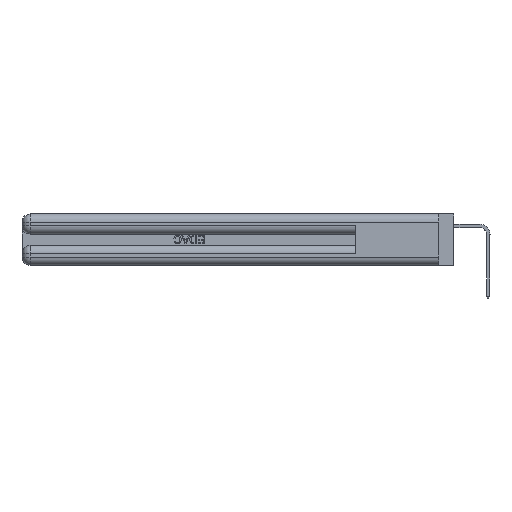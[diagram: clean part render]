
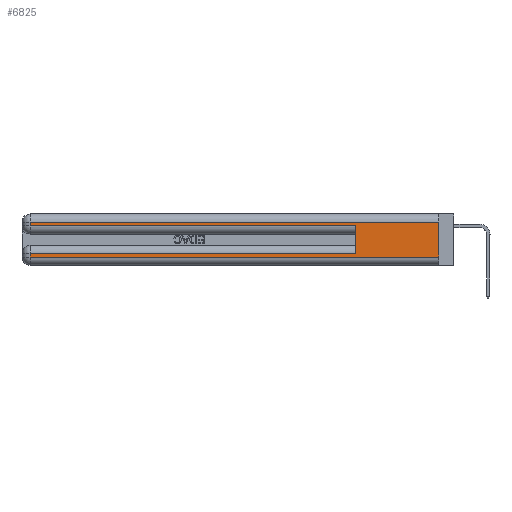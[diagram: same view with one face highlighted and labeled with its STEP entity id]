
A CAD part, left-side view. The second image highlights one B-rep face of the part: STEP entity #6825.
In plain terms, the highlighted planar face has unit normal (-1, 0, 0).
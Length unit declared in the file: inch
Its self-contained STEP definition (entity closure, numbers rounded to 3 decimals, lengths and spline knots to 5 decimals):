
#51 = CARTESIAN_POINT ( 'NONE',  ( 0., 0., 0.31 ) ) ;
#1220 = ORIENTED_EDGE ( 'NONE', *, *, #40643, .T. ) ;
#1501 = LINE ( 'NONE', #16280, #30287 ) ;
#1597 = VECTOR ( 'NONE', #37832, 39.37008 ) ;
#2039 = EDGE_CURVE ( 'NONE', #19701, #25702, #11269, .T. ) ;
#2242 = FACE_OUTER_BOUND ( 'NONE', #19617, .T. ) ;
#2839 = ORIENTED_EDGE ( 'NONE', *, *, #21379, .F. ) ;
#3561 = VERTEX_POINT ( 'NONE', #28904 ) ;
#5607 = PLANE ( 'NONE',  #5820 ) ;
#5661 = LINE ( 'NONE', #15015, #25240 ) ;
#5781 = VECTOR ( 'NONE', #19699, 39.37008 ) ;
#5820 = AXIS2_PLACEMENT_3D ( 'NONE', #48293, #32975, #9551 ) ;
#6825 = ADVANCED_FACE ( 'NONE', ( #2242 ), #5607, .F. ) ;
#7211 = CARTESIAN_POINT ( 'NONE',  ( 0., 0.6, 0.285 ) ) ;
#9551 = DIRECTION ( 'NONE',  ( 0., 0., -1. ) ) ;
#9796 = ORIENTED_EDGE ( 'NONE', *, *, #33480, .T. ) ;
#11269 = LINE ( 'NONE', #28252, #21680 ) ;
#13544 = LINE ( 'NONE', #34298, #42243 ) ;
#14142 = VECTOR ( 'NONE', #47552, 39.37008 ) ;
#15015 = CARTESIAN_POINT ( 'NONE',  ( 0., 2.94, 0.37 ) ) ;
#15180 = EDGE_CURVE ( 'NONE', #19701, #49928, #44286, .T. ) ;
#16280 = CARTESIAN_POINT ( 'NONE',  ( 0., 2.94, 0.37 ) ) ;
#18287 = ORIENTED_EDGE ( 'NONE', *, *, #47482, .T. ) ;
#18958 = DIRECTION ( 'NONE',  ( 0., 0., -1. ) ) ;
#19617 = EDGE_LOOP ( 'NONE', ( #2839, #1220, #26896, #18287, #28642, #39862, #22399, #9796 ) ) ;
#19699 = DIRECTION ( 'NONE',  ( 0., 0., -1. ) ) ;
#19701 = VERTEX_POINT ( 'NONE', #23728 ) ;
#20630 = CARTESIAN_POINT ( 'NONE',  ( 0., 0., 0.31 ) ) ;
#21379 = EDGE_CURVE ( 'NONE', #25191, #44203, #25366, .T. ) ;
#21680 = VECTOR ( 'NONE', #47673, 39.37008 ) ;
#21841 = DIRECTION ( 'NONE',  ( 0., 1., 0. ) ) ;
#22399 = ORIENTED_EDGE ( 'NONE', *, *, #30893, .T. ) ;
#23728 = CARTESIAN_POINT ( 'NONE',  ( 0., 0.6, 0.085 ) ) ;
#25191 = VERTEX_POINT ( 'NONE', #51 ) ;
#25240 = VECTOR ( 'NONE', #18958, 39.37008 ) ;
#25366 = LINE ( 'NONE', #43038, #5781 ) ;
#25702 = VERTEX_POINT ( 'NONE', #7211 ) ;
#26607 = DIRECTION ( 'NONE',  ( 0., -1., 0. ) ) ;
#26896 = ORIENTED_EDGE ( 'NONE', *, *, #31851, .T. ) ;
#28037 = DIRECTION ( 'NONE',  ( 0., 0., -1. ) ) ;
#28252 = CARTESIAN_POINT ( 'NONE',  ( 0., 0.6, 0.145 ) ) ;
#28642 = ORIENTED_EDGE ( 'NONE', *, *, #2039, .F. ) ;
#28904 = CARTESIAN_POINT ( 'NONE',  ( 0., 2.94, 0.06 ) ) ;
#30287 = VECTOR ( 'NONE', #28037, 39.37008 ) ;
#30893 = EDGE_CURVE ( 'NONE', #49928, #3561, #1501, .T. ) ;
#31851 = EDGE_CURVE ( 'NONE', #49597, #37296, #5661, .T. ) ;
#32461 = LINE ( 'NONE', #20630, #14142 ) ;
#32691 = VECTOR ( 'NONE', #21841, 39.37008 ) ;
#32975 = DIRECTION ( 'NONE',  ( 1., 0., 0. ) ) ;
#33480 = EDGE_CURVE ( 'NONE', #3561, #44203, #13544, .T. ) ;
#34298 = CARTESIAN_POINT ( 'NONE',  ( 0., 0., 0.06 ) ) ;
#35158 = CARTESIAN_POINT ( 'NONE',  ( 0., 0., 0.06 ) ) ;
#37296 = VERTEX_POINT ( 'NONE', #37383 ) ;
#37375 = CARTESIAN_POINT ( 'NONE',  ( 0., 0., 0.085 ) ) ;
#37383 = CARTESIAN_POINT ( 'NONE',  ( 0., 2.94, 0.285 ) ) ;
#37832 = DIRECTION ( 'NONE',  ( 0., -1., 0. ) ) ;
#38710 = CARTESIAN_POINT ( 'NONE',  ( 0., 2.94, 0.31 ) ) ;
#39862 = ORIENTED_EDGE ( 'NONE', *, *, #15180, .T. ) ;
#40554 = CARTESIAN_POINT ( 'NONE',  ( 0., 2.94, 0.085 ) ) ;
#40643 = EDGE_CURVE ( 'NONE', #25191, #49597, #32461, .T. ) ;
#41765 = CARTESIAN_POINT ( 'NONE',  ( 0., 0., 0.285 ) ) ;
#42243 = VECTOR ( 'NONE', #26607, 39.37008 ) ;
#43038 = CARTESIAN_POINT ( 'NONE',  ( 0., 0., 0.37 ) ) ;
#43143 = LINE ( 'NONE', #41765, #1597 ) ;
#44203 = VERTEX_POINT ( 'NONE', #35158 ) ;
#44286 = LINE ( 'NONE', #37375, #32691 ) ;
#47482 = EDGE_CURVE ( 'NONE', #37296, #25702, #43143, .T. ) ;
#47552 = DIRECTION ( 'NONE',  ( 0., 1., 0. ) ) ;
#47673 = DIRECTION ( 'NONE',  ( 0., 0., 1. ) ) ;
#48293 = CARTESIAN_POINT ( 'NONE',  ( 0., 0., 0.37 ) ) ;
#49597 = VERTEX_POINT ( 'NONE', #38710 ) ;
#49928 = VERTEX_POINT ( 'NONE', #40554 ) ;
